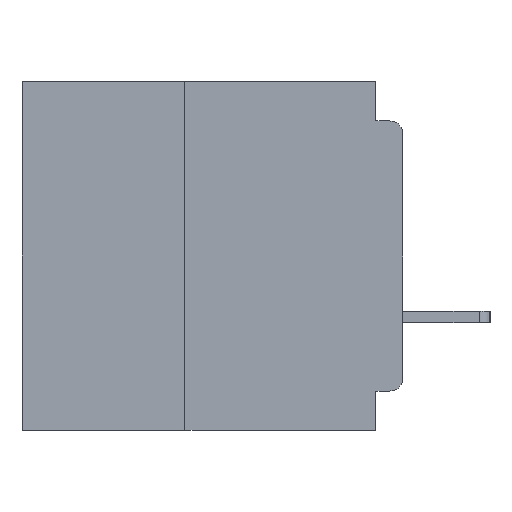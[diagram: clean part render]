
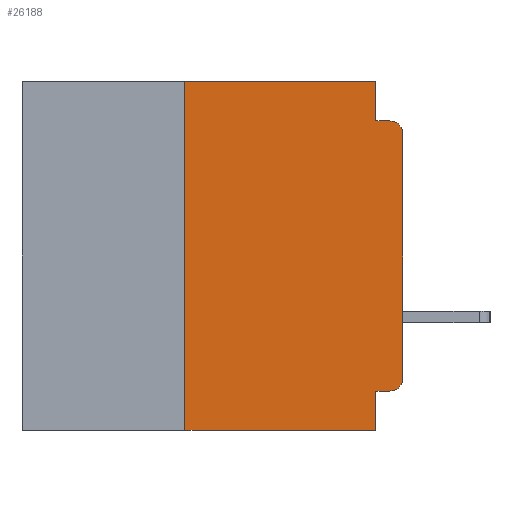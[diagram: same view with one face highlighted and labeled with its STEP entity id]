
A CAD part, left-side view. The second image highlights one B-rep face of the part: STEP entity #26188.
In plain terms, the highlighted planar face has unit normal (-1, 0, 0).
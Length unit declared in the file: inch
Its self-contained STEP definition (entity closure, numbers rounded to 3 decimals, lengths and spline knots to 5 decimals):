
#53 = ORIENTED_EDGE ( 'NONE', *, *, #11561, .F. ) ;
#331 = FACE_OUTER_BOUND ( 'NONE', #36567, .T. ) ;
#848 = DIRECTION ( 'NONE',  ( 0., 0., 1. ) ) ;
#2685 = DIRECTION ( 'NONE',  ( 0., 0., -1. ) ) ;
#3295 = VECTOR ( 'NONE', #8351, 39.37008 ) ;
#3889 = VERTEX_POINT ( 'NONE', #21884 ) ;
#4551 = VERTEX_POINT ( 'NONE', #23281 ) ;
#4775 = VERTEX_POINT ( 'NONE', #8353 ) ;
#5279 = VECTOR ( 'NONE', #22728, 39.37008 ) ;
#5470 = ORIENTED_EDGE ( 'NONE', *, *, #38982, .F. ) ;
#7451 = ORIENTED_EDGE ( 'NONE', *, *, #21665, .T. ) ;
#7551 = DIRECTION ( 'NONE',  ( 0., 0., -1. ) ) ;
#7601 = VECTOR ( 'NONE', #12244, 39.37008 ) ;
#7899 = ORIENTED_EDGE ( 'NONE', *, *, #10056, .F. ) ;
#8351 = DIRECTION ( 'NONE',  ( 0., 1., 0. ) ) ;
#8353 = CARTESIAN_POINT ( 'NONE',  ( 0., 0.031, -0.355 ) ) ;
#8434 = ORIENTED_EDGE ( 'NONE', *, *, #36925, .F. ) ;
#8552 = LINE ( 'NONE', #9096, #7601 ) ;
#9096 = CARTESIAN_POINT ( 'NONE',  ( 0., 0.031, -0.4 ) ) ;
#10056 = EDGE_CURVE ( 'NONE', #14084, #35176, #38547, .T. ) ;
#10073 = DIRECTION ( 'NONE',  ( 0., -1., 0. ) ) ;
#10498 = EDGE_CURVE ( 'NONE', #23159, #4551, #15464, .T. ) ;
#10769 = CIRCLE ( 'NONE', #35184, 0.015 ) ;
#10785 = VERTEX_POINT ( 'NONE', #14459 ) ;
#10983 = VECTOR ( 'NONE', #33348, 39.37008 ) ;
#11081 = PLANE ( 'NONE',  #33084 ) ;
#11356 = CARTESIAN_POINT ( 'NONE',  ( 0., 0.015, -0.06 ) ) ;
#11561 = EDGE_CURVE ( 'NONE', #4775, #31556, #8552, .T. ) ;
#12244 = DIRECTION ( 'NONE',  ( 0., 0., -1. ) ) ;
#13210 = CARTESIAN_POINT ( 'NONE',  ( 0., 0., -0.045 ) ) ;
#14006 = EDGE_CURVE ( 'NONE', #35176, #24620, #28663, .T. ) ;
#14084 = VERTEX_POINT ( 'NONE', #35760 ) ;
#14185 = DIRECTION ( 'NONE',  ( 0., 0., -1. ) ) ;
#14459 = CARTESIAN_POINT ( 'NONE',  ( 0., 0.015, -0.045 ) ) ;
#14461 = DIRECTION ( 'NONE',  ( 0., 0., -1. ) ) ;
#14671 = ORIENTED_EDGE ( 'NONE', *, *, #25674, .F. ) ;
#14850 = VECTOR ( 'NONE', #848, 39.37008 ) ;
#15464 = LINE ( 'NONE', #28381, #23622 ) ;
#18098 = CARTESIAN_POINT ( 'NONE',  ( 0., 0.031, 0. ) ) ;
#18739 = CARTESIAN_POINT ( 'NONE',  ( 0., 0., -0.34 ) ) ;
#18948 = CARTESIAN_POINT ( 'NONE',  ( 0., 0.031, -0.4 ) ) ;
#20030 = AXIS2_PLACEMENT_3D ( 'NONE', #11356, #32917, #14461 ) ;
#20527 = ORIENTED_EDGE ( 'NONE', *, *, #35800, .T. ) ;
#20922 = ORIENTED_EDGE ( 'NONE', *, *, #30969, .T. ) ;
#21054 = VERTEX_POINT ( 'NONE', #33401 ) ;
#21282 = DIRECTION ( 'NONE',  ( -1., 0., 0. ) ) ;
#21432 = ORIENTED_EDGE ( 'NONE', *, *, #14006, .F. ) ;
#21665 = EDGE_CURVE ( 'NONE', #3889, #31556, #27381, .T. ) ;
#21884 = CARTESIAN_POINT ( 'NONE',  ( 0., 0.25, -0.4 ) ) ;
#22728 = DIRECTION ( 'NONE',  ( 0., -1., 0. ) ) ;
#23159 = VERTEX_POINT ( 'NONE', #18739 ) ;
#23281 = CARTESIAN_POINT ( 'NONE',  ( 0., 0., -0.06 ) ) ;
#23331 = CIRCLE ( 'NONE', #20030, 0.015 ) ;
#23622 = VECTOR ( 'NONE', #31471, 39.37008 ) ;
#24620 = VERTEX_POINT ( 'NONE', #29579 ) ;
#25674 = EDGE_CURVE ( 'NONE', #24620, #10785, #37213, .T. ) ;
#25691 = CARTESIAN_POINT ( 'NONE',  ( 0., 0.25, -0.4 ) ) ;
#26188 = ADVANCED_FACE ( 'NONE', ( #331 ), #11081, .F. ) ;
#27381 = LINE ( 'NONE', #39632, #10983 ) ;
#28069 = VECTOR ( 'NONE', #10073, 39.37008 ) ;
#28381 = CARTESIAN_POINT ( 'NONE',  ( 0., 0., 0. ) ) ;
#28663 = LINE ( 'NONE', #29166, #35884 ) ;
#29166 = CARTESIAN_POINT ( 'NONE',  ( 0., 0.031, 0. ) ) ;
#29579 = CARTESIAN_POINT ( 'NONE',  ( 0., 0.031, -0.045 ) ) ;
#30969 = EDGE_CURVE ( 'NONE', #4551, #10785, #23331, .T. ) ;
#31262 = LINE ( 'NONE', #25691, #14850 ) ;
#31471 = DIRECTION ( 'NONE',  ( 0., 0., 1. ) ) ;
#31556 = VERTEX_POINT ( 'NONE', #18948 ) ;
#32502 = CARTESIAN_POINT ( 'NONE',  ( 0., 0.437, 0. ) ) ;
#32635 = DIRECTION ( 'NONE',  ( 1., 0., 0. ) ) ;
#32917 = DIRECTION ( 'NONE',  ( -1., 0., 0. ) ) ;
#32927 = CARTESIAN_POINT ( 'NONE',  ( 0., 0., -0.355 ) ) ;
#33084 = AXIS2_PLACEMENT_3D ( 'NONE', #32502, #32635, #14185 ) ;
#33348 = DIRECTION ( 'NONE',  ( 0., -1., 0. ) ) ;
#33401 = CARTESIAN_POINT ( 'NONE',  ( 0., 0.015, -0.355 ) ) ;
#35012 = CARTESIAN_POINT ( 'NONE',  ( 0., 0.437, 0. ) ) ;
#35176 = VERTEX_POINT ( 'NONE', #18098 ) ;
#35184 = AXIS2_PLACEMENT_3D ( 'NONE', #39700, #21282, #2685 ) ;
#35760 = CARTESIAN_POINT ( 'NONE',  ( 0., 0.25, 0. ) ) ;
#35800 = EDGE_CURVE ( 'NONE', #21054, #23159, #10769, .T. ) ;
#35884 = VECTOR ( 'NONE', #7551, 39.37008 ) ;
#36235 = LINE ( 'NONE', #32927, #3295 ) ;
#36393 = ORIENTED_EDGE ( 'NONE', *, *, #10498, .T. ) ;
#36567 = EDGE_LOOP ( 'NONE', ( #36393, #20922, #14671, #21432, #7899, #5470, #7451, #53, #8434, #20527 ) ) ;
#36925 = EDGE_CURVE ( 'NONE', #21054, #4775, #36235, .T. ) ;
#37213 = LINE ( 'NONE', #13210, #28069 ) ;
#38547 = LINE ( 'NONE', #35012, #5279 ) ;
#38982 = EDGE_CURVE ( 'NONE', #3889, #14084, #31262, .T. ) ;
#39632 = CARTESIAN_POINT ( 'NONE',  ( 0., 0.437, -0.4 ) ) ;
#39700 = CARTESIAN_POINT ( 'NONE',  ( 0., 0.015, -0.34 ) ) ;
